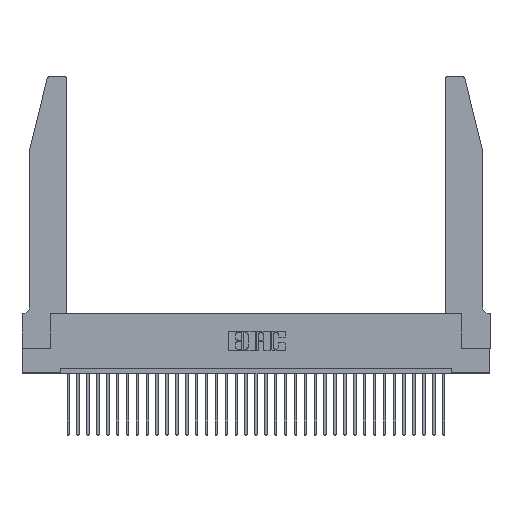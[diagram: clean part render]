
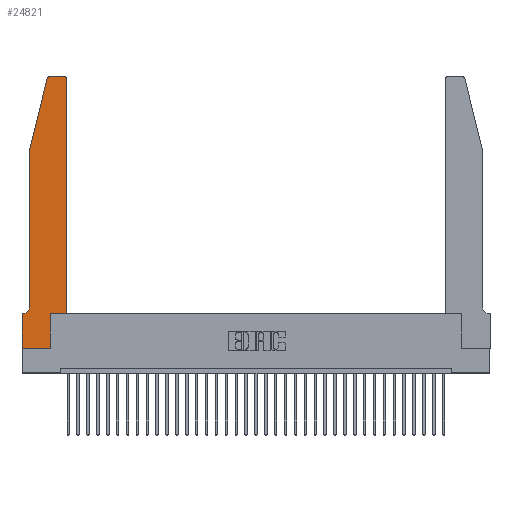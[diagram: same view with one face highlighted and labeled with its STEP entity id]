
A CAD part, top view. The second image highlights one B-rep face of the part: STEP entity #24821.
In plain terms, the highlighted planar face has unit normal (0, 0, 1).
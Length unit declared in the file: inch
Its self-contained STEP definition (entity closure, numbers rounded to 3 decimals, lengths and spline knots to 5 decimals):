
#112 = DIRECTION ( 'NONE',  ( 1., 0., 0. ) ) ;
#648 = DIRECTION ( 'NONE',  ( -1., 0., 0. ) ) ;
#777 = ORIENTED_EDGE ( 'NONE', *, *, #29452, .T. ) ;
#897 = VECTOR ( 'NONE', #10798, 39.37008 ) ;
#1386 = ORIENTED_EDGE ( 'NONE', *, *, #6817, .T. ) ;
#1668 = EDGE_CURVE ( 'NONE', #14206, #13051, #23606, .T. ) ;
#1881 = VERTEX_POINT ( 'NONE', #25079 ) ;
#2011 = DIRECTION ( 'NONE',  ( 1., 0., 0. ) ) ;
#2995 = AXIS2_PLACEMENT_3D ( 'NONE', #6807, #17303, #11939 ) ;
#3028 = ORIENTED_EDGE ( 'NONE', *, *, #15502, .T. ) ;
#3418 = LINE ( 'NONE', #34422, #897 ) ;
#3746 = DIRECTION ( 'NONE',  ( -0.239, -0.971, 0. ) ) ;
#4160 = VERTEX_POINT ( 'NONE', #20459 ) ;
#4239 = CARTESIAN_POINT ( 'NONE',  ( 0.0755, 2., 0.37 ) ) ;
#4259 = EDGE_CURVE ( 'NONE', #4160, #14206, #12519, .T. ) ;
#4756 = DIRECTION ( 'NONE',  ( 0., -1., 0. ) ) ;
#5419 = EDGE_CURVE ( 'NONE', #1881, #21374, #29093, .T. ) ;
#6199 = VECTOR ( 'NONE', #14339, 39.37008 ) ;
#6807 = CARTESIAN_POINT ( 'NONE',  ( 0.0055, 0.42, 0.37 ) ) ;
#6817 = EDGE_CURVE ( 'NONE', #21374, #25695, #15998, .T. ) ;
#6936 = CARTESIAN_POINT ( 'NONE',  ( 0.0755, 0.42, 0.37 ) ) ;
#6977 = EDGE_CURVE ( 'NONE', #23801, #13365, #32748, .T. ) ;
#7337 = CARTESIAN_POINT ( 'NONE',  ( 0.4205, 2.75, 0.37 ) ) ;
#7845 = CARTESIAN_POINT ( 'NONE',  ( 0.4505, 0.35, 0.37 ) ) ;
#7889 = CIRCLE ( 'NONE', #2995, 0.07 ) ;
#8150 = VECTOR ( 'NONE', #4756, 39.37008 ) ;
#8277 = ORIENTED_EDGE ( 'NONE', *, *, #1668, .T. ) ;
#8349 = EDGE_CURVE ( 'NONE', #13365, #13025, #24286, .T. ) ;
#9166 = ORIENTED_EDGE ( 'NONE', *, *, #21925, .T. ) ;
#9408 = VECTOR ( 'NONE', #26720, 39.37008 ) ;
#10414 = ORIENTED_EDGE ( 'NONE', *, *, #5419, .T. ) ;
#10798 = DIRECTION ( 'NONE',  ( 0., -1., 0. ) ) ;
#11311 = VECTOR ( 'NONE', #112, 39.37008 ) ;
#11626 = CARTESIAN_POINT ( 'NONE',  ( 0.4205, 2.72, 0.37 ) ) ;
#11805 = CARTESIAN_POINT ( 'NONE',  ( 0.2865, 0.35, 0.37 ) ) ;
#11939 = DIRECTION ( 'NONE',  ( -1., 0., 0. ) ) ;
#12118 = LINE ( 'NONE', #4239, #18355 ) ;
#12519 = LINE ( 'NONE', #11805, #22576 ) ;
#13025 = VERTEX_POINT ( 'NONE', #27478 ) ;
#13051 = VERTEX_POINT ( 'NONE', #27598 ) ;
#13231 = CARTESIAN_POINT ( 'NONE',  ( 0.4505, 2.72, 0.37 ) ) ;
#13272 = CARTESIAN_POINT ( 'NONE',  ( 0.4505, 0.35, 0.37 ) ) ;
#13365 = VERTEX_POINT ( 'NONE', #7337 ) ;
#13674 = ORIENTED_EDGE ( 'NONE', *, *, #31646, .T. ) ;
#14206 = VERTEX_POINT ( 'NONE', #21062 ) ;
#14339 = DIRECTION ( 'NONE',  ( -1., 0., 0. ) ) ;
#15502 = EDGE_CURVE ( 'NONE', #20281, #24496, #12118, .T. ) ;
#15687 = CIRCLE ( 'NONE', #30111, 0.03 ) ;
#15791 = CARTESIAN_POINT ( 'NONE',  ( 0., 0., 0.37 ) ) ;
#15998 = LINE ( 'NONE', #20568, #8150 ) ;
#16866 = CARTESIAN_POINT ( 'NONE',  ( 0.284, 2.72, 0.37 ) ) ;
#17170 = ORIENTED_EDGE ( 'NONE', *, *, #24536, .T. ) ;
#17300 = CARTESIAN_POINT ( 'NONE',  ( 0.25487, 2.72718, 0.37 ) ) ;
#17303 = DIRECTION ( 'NONE',  ( 0., 0., -1. ) ) ;
#17681 = PLANE ( 'NONE',  #19643 ) ;
#17981 = EDGE_CURVE ( 'NONE', #13051, #23801, #20738, .T. ) ;
#18008 = VECTOR ( 'NONE', #648, 39.37008 ) ;
#18355 = VECTOR ( 'NONE', #3746, 39.37008 ) ;
#18683 = CARTESIAN_POINT ( 'NONE',  ( 0.2605, 2.75, 0.37 ) ) ;
#18955 = ORIENTED_EDGE ( 'NONE', *, *, #6977, .T. ) ;
#19201 = EDGE_LOOP ( 'NONE', ( #32109, #17170, #3028, #777, #13674, #10414, #1386, #9166, #29861, #8277, #27033, #18955 ) ) ;
#19344 = DIRECTION ( 'NONE',  ( 0., 0., 1. ) ) ;
#19643 = AXIS2_PLACEMENT_3D ( 'NONE', #31401, #28665, #2011 ) ;
#20281 = VERTEX_POINT ( 'NONE', #17300 ) ;
#20459 = CARTESIAN_POINT ( 'NONE',  ( 0.2865, 0., 0.37 ) ) ;
#20568 = CARTESIAN_POINT ( 'NONE',  ( 0., 0., 0.37 ) ) ;
#20738 = LINE ( 'NONE', #7845, #24049 ) ;
#21062 = CARTESIAN_POINT ( 'NONE',  ( 0.2865, 0.35, 0.37 ) ) ;
#21374 = VERTEX_POINT ( 'NONE', #25153 ) ;
#21925 = EDGE_CURVE ( 'NONE', #25695, #4160, #22664, .T. ) ;
#22189 = AXIS2_PLACEMENT_3D ( 'NONE', #11626, #30194, #30078 ) ;
#22576 = VECTOR ( 'NONE', #24902, 39.37008 ) ;
#22664 = LINE ( 'NONE', #15791, #11311 ) ;
#23274 = FACE_OUTER_BOUND ( 'NONE', #19201, .T. ) ;
#23606 = LINE ( 'NONE', #13272, #9408 ) ;
#23801 = VERTEX_POINT ( 'NONE', #13231 ) ;
#24049 = VECTOR ( 'NONE', #29127, 39.37008 ) ;
#24286 = LINE ( 'NONE', #18683, #18008 ) ;
#24496 = VERTEX_POINT ( 'NONE', #29967 ) ;
#24536 = EDGE_CURVE ( 'NONE', #13025, #20281, #15687, .T. ) ;
#24821 = ADVANCED_FACE ( 'NONE', ( #23274 ), #17681, .T. ) ;
#24902 = DIRECTION ( 'NONE',  ( 0., 1., 0. ) ) ;
#24905 = VERTEX_POINT ( 'NONE', #6936 ) ;
#25079 = CARTESIAN_POINT ( 'NONE',  ( 0.0055, 0.35, 0.37 ) ) ;
#25153 = CARTESIAN_POINT ( 'NONE',  ( 0., 0.35, 0.37 ) ) ;
#25695 = VERTEX_POINT ( 'NONE', #29492 ) ;
#26720 = DIRECTION ( 'NONE',  ( 1., 0., 0. ) ) ;
#27033 = ORIENTED_EDGE ( 'NONE', *, *, #17981, .T. ) ;
#27478 = CARTESIAN_POINT ( 'NONE',  ( 0.284, 2.75, 0.37 ) ) ;
#27598 = CARTESIAN_POINT ( 'NONE',  ( 0.4505, 0.35, 0.37 ) ) ;
#27648 = DIRECTION ( 'NONE',  ( 1., 0., 0. ) ) ;
#28665 = DIRECTION ( 'NONE',  ( 0., 0., 1. ) ) ;
#29093 = LINE ( 'NONE', #33201, #6199 ) ;
#29127 = DIRECTION ( 'NONE',  ( 0., 1., 0. ) ) ;
#29452 = EDGE_CURVE ( 'NONE', #24496, #24905, #3418, .T. ) ;
#29492 = CARTESIAN_POINT ( 'NONE',  ( 0., 0., 0.37 ) ) ;
#29861 = ORIENTED_EDGE ( 'NONE', *, *, #4259, .T. ) ;
#29967 = CARTESIAN_POINT ( 'NONE',  ( 0.0755, 2., 0.37 ) ) ;
#30078 = DIRECTION ( 'NONE',  ( 1., 0., 0. ) ) ;
#30111 = AXIS2_PLACEMENT_3D ( 'NONE', #16866, #19344, #27648 ) ;
#30194 = DIRECTION ( 'NONE',  ( 0., 0., 1. ) ) ;
#31401 = CARTESIAN_POINT ( 'NONE',  ( 0., 0.35, 0.37 ) ) ;
#31646 = EDGE_CURVE ( 'NONE', #24905, #1881, #7889, .T. ) ;
#32109 = ORIENTED_EDGE ( 'NONE', *, *, #8349, .T. ) ;
#32748 = CIRCLE ( 'NONE', #22189, 0.03 ) ;
#33201 = CARTESIAN_POINT ( 'NONE',  ( 0.0755, 0.35, 0.37 ) ) ;
#34422 = CARTESIAN_POINT ( 'NONE',  ( 0.0755, 2., 0.37 ) ) ;
